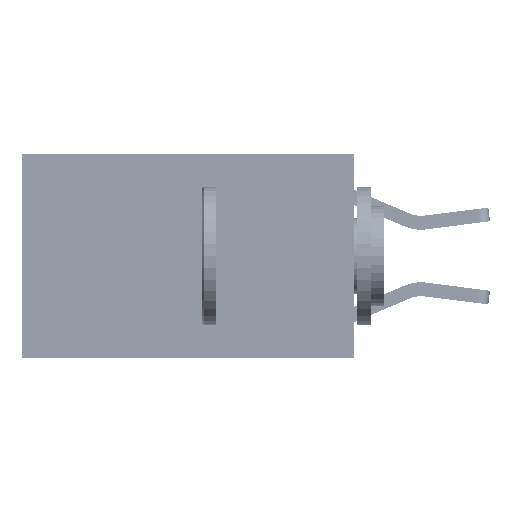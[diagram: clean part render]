
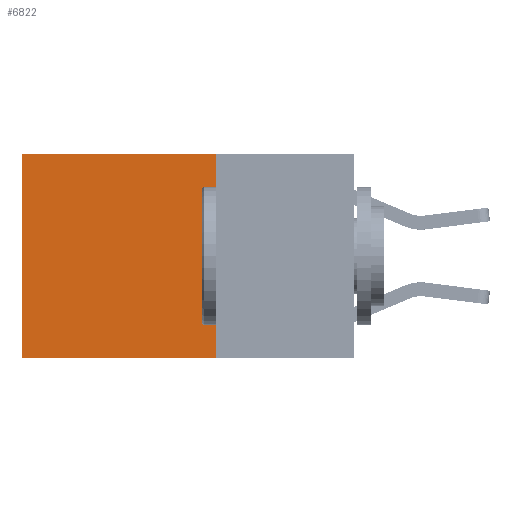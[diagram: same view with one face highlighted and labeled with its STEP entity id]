
A CAD part, left-side view. The second image highlights one B-rep face of the part: STEP entity #6822.
In plain terms, the highlighted planar face has unit normal (-1, 0, 0).
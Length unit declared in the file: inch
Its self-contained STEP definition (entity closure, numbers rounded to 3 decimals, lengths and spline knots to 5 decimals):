
#78 = VECTOR ( 'NONE', #1206, 39.37008 ) ;
#1206 = DIRECTION ( 'NONE',  ( 0., 0., -1. ) ) ;
#1277 = EDGE_CURVE ( 'NONE', #10082, #5786, #28401, .T. ) ;
#1281 = CARTESIAN_POINT ( 'NONE',  ( 0.2625, 0.25, -0.37 ) ) ;
#1703 = VERTEX_POINT ( 'NONE', #19802 ) ;
#2399 = EDGE_CURVE ( 'NONE', #1703, #10082, #4490, .T. ) ;
#3760 = ORIENTED_EDGE ( 'NONE', *, *, #17101, .F. ) ;
#4044 = CARTESIAN_POINT ( 'NONE',  ( 0.2625, 0.25, 0. ) ) ;
#4490 = LINE ( 'NONE', #14377, #29766 ) ;
#4825 = CARTESIAN_POINT ( 'NONE',  ( 0.2625, 0.25, 0. ) ) ;
#5555 = EDGE_LOOP ( 'NONE', ( #28966, #31636, #3760, #14461 ) ) ;
#5786 = VERTEX_POINT ( 'NONE', #21457 ) ;
#5982 = DIRECTION ( 'NONE',  ( 1., 0., 0. ) ) ;
#6105 = CARTESIAN_POINT ( 'NONE',  ( 0.2625, 0.25, -0.37 ) ) ;
#6404 = AXIS2_PLACEMENT_3D ( 'NONE', #4044, #5982, #15873 ) ;
#6466 = FACE_OUTER_BOUND ( 'NONE', #5555, .T. ) ;
#6822 = ADVANCED_FACE ( 'NONE', ( #6466 ), #26229, .F. ) ;
#7147 = VECTOR ( 'NONE', #24599, 39.37008 ) ;
#7888 = LINE ( 'NONE', #4825, #7147 ) ;
#8628 = VERTEX_POINT ( 'NONE', #6105 ) ;
#10082 = VERTEX_POINT ( 'NONE', #15347 ) ;
#12563 = EDGE_CURVE ( 'NONE', #8628, #5786, #21046, .T. ) ;
#14377 = CARTESIAN_POINT ( 'NONE',  ( 0.2625, 0.25, 0. ) ) ;
#14461 = ORIENTED_EDGE ( 'NONE', *, *, #2399, .T. ) ;
#15347 = CARTESIAN_POINT ( 'NONE',  ( 0.2625, 0.6, 0. ) ) ;
#15873 = DIRECTION ( 'NONE',  ( 0., 0., -1. ) ) ;
#17101 = EDGE_CURVE ( 'NONE', #1703, #8628, #7888, .T. ) ;
#19257 = DIRECTION ( 'NONE',  ( 0., 1., 0. ) ) ;
#19802 = CARTESIAN_POINT ( 'NONE',  ( 0.2625, 0.25, 0. ) ) ;
#21046 = LINE ( 'NONE', #1281, #30356 ) ;
#21457 = CARTESIAN_POINT ( 'NONE',  ( 0.2625, 0.6, -0.37 ) ) ;
#24258 = DIRECTION ( 'NONE',  ( 0., 1., 0. ) ) ;
#24599 = DIRECTION ( 'NONE',  ( 0., 0., -1. ) ) ;
#26229 = PLANE ( 'NONE',  #6404 ) ;
#28401 = LINE ( 'NONE', #31312, #78 ) ;
#28966 = ORIENTED_EDGE ( 'NONE', *, *, #1277, .T. ) ;
#29766 = VECTOR ( 'NONE', #24258, 39.37008 ) ;
#30356 = VECTOR ( 'NONE', #19257, 39.37008 ) ;
#31312 = CARTESIAN_POINT ( 'NONE',  ( 0.2625, 0.6, 0. ) ) ;
#31636 = ORIENTED_EDGE ( 'NONE', *, *, #12563, .F. ) ;
